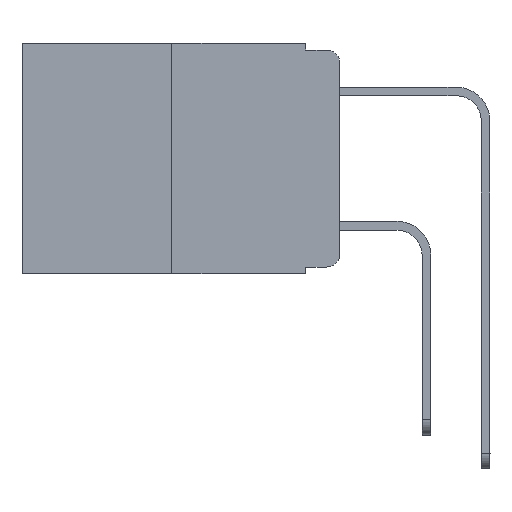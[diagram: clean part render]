
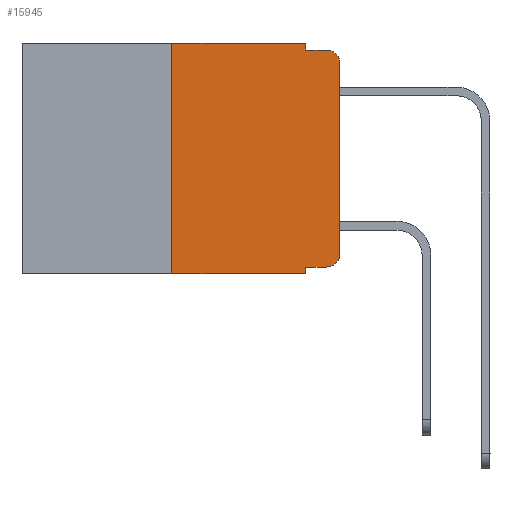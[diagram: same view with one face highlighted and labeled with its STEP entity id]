
A CAD part, left-side view. The second image highlights one B-rep face of the part: STEP entity #15945.
In plain terms, the highlighted planar face has unit normal (-1, 0, 0).
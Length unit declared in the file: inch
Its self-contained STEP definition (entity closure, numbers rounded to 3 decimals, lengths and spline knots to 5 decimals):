
#130 = VECTOR ( 'NONE', #8051, 39.37008 ) ;
#310 = ORIENTED_EDGE ( 'NONE', *, *, #6966, .T. ) ;
#363 = CARTESIAN_POINT ( 'NONE',  ( 0., 0., 0. ) ) ;
#552 = CARTESIAN_POINT ( 'NONE',  ( 0., 0.25, -0.343 ) ) ;
#640 = CARTESIAN_POINT ( 'NONE',  ( 0., 0.473, 0. ) ) ;
#662 = LINE ( 'NONE', #10816, #15736 ) ;
#1404 = VERTEX_POINT ( 'NONE', #552 ) ;
#1606 = VERTEX_POINT ( 'NONE', #12505 ) ;
#1628 = VECTOR ( 'NONE', #15412, 39.37008 ) ;
#1970 = LINE ( 'NONE', #9194, #6161 ) ;
#2006 = VERTEX_POINT ( 'NONE', #8278 ) ;
#2030 = ORIENTED_EDGE ( 'NONE', *, *, #8877, .F. ) ;
#2296 = DIRECTION ( 'NONE',  ( 1., 0., 0. ) ) ;
#2863 = ORIENTED_EDGE ( 'NONE', *, *, #17228, .F. ) ;
#2881 = VECTOR ( 'NONE', #17953, 39.37008 ) ;
#3000 = EDGE_CURVE ( 'NONE', #16953, #4364, #6071, .T. ) ;
#3018 = DIRECTION ( 'NONE',  ( 0., 0., 1. ) ) ;
#3477 = LINE ( 'NONE', #640, #3752 ) ;
#3718 = AXIS2_PLACEMENT_3D ( 'NONE', #7315, #15811, #14385 ) ;
#3752 = VECTOR ( 'NONE', #10371, 39.37008 ) ;
#3949 = VECTOR ( 'NONE', #8951, 39.37008 ) ;
#4364 = VERTEX_POINT ( 'NONE', #15149 ) ;
#4545 = CIRCLE ( 'NONE', #10470, 0.02 ) ;
#4652 = CARTESIAN_POINT ( 'NONE',  ( 0., 0.25, 0. ) ) ;
#4974 = ORIENTED_EDGE ( 'NONE', *, *, #6975, .T. ) ;
#5080 = LINE ( 'NONE', #8145, #130 ) ;
#5528 = ORIENTED_EDGE ( 'NONE', *, *, #12385, .T. ) ;
#6071 = LINE ( 'NONE', #363, #14674 ) ;
#6157 = CARTESIAN_POINT ( 'NONE',  ( 0., 0.051, -0.333 ) ) ;
#6161 = VECTOR ( 'NONE', #7621, 39.37008 ) ;
#6610 = LINE ( 'NONE', #12227, #2881 ) ;
#6828 = CARTESIAN_POINT ( 'NONE',  ( 0., 0., -0.313 ) ) ;
#6966 = EDGE_CURVE ( 'NONE', #4364, #10477, #4545, .T. ) ;
#6975 = EDGE_CURVE ( 'NONE', #1404, #7607, #5080, .T. ) ;
#7315 = CARTESIAN_POINT ( 'NONE',  ( 0., 0.02, -0.313 ) ) ;
#7607 = VERTEX_POINT ( 'NONE', #14930 ) ;
#7621 = DIRECTION ( 'NONE',  ( 0., -1., 0. ) ) ;
#8051 = DIRECTION ( 'NONE',  ( 0., -1., 0. ) ) ;
#8145 = CARTESIAN_POINT ( 'NONE',  ( 0., 0.473, -0.343 ) ) ;
#8229 = FACE_OUTER_BOUND ( 'NONE', #14494, .T. ) ;
#8278 = CARTESIAN_POINT ( 'NONE',  ( 0., 0.051, -0.01 ) ) ;
#8298 = VERTEX_POINT ( 'NONE', #16605 ) ;
#8877 = EDGE_CURVE ( 'NONE', #1606, #7607, #15326, .T. ) ;
#8951 = DIRECTION ( 'NONE',  ( 0., -1., 0. ) ) ;
#9020 = EDGE_CURVE ( 'NONE', #1606, #12892, #13046, .T. ) ;
#9194 = CARTESIAN_POINT ( 'NONE',  ( 0., 0.051, -0.01 ) ) ;
#10232 = ORIENTED_EDGE ( 'NONE', *, *, #11311, .F. ) ;
#10371 = DIRECTION ( 'NONE',  ( 0., -1., 0. ) ) ;
#10470 = AXIS2_PLACEMENT_3D ( 'NONE', #15003, #16252, #17818 ) ;
#10477 = VERTEX_POINT ( 'NONE', #16560 ) ;
#10610 = VERTEX_POINT ( 'NONE', #4652 ) ;
#10810 = PLANE ( 'NONE',  #15209 ) ;
#10816 = CARTESIAN_POINT ( 'NONE',  ( 0., 0.25, 0. ) ) ;
#11289 = ORIENTED_EDGE ( 'NONE', *, *, #17674, .F. ) ;
#11311 = EDGE_CURVE ( 'NONE', #1404, #10610, #662, .T. ) ;
#11537 = ORIENTED_EDGE ( 'NONE', *, *, #3000, .T. ) ;
#12227 = CARTESIAN_POINT ( 'NONE',  ( 0., 0.051, 0. ) ) ;
#12385 = EDGE_CURVE ( 'NONE', #12892, #16953, #16034, .T. ) ;
#12505 = CARTESIAN_POINT ( 'NONE',  ( 0., 0.051, -0.333 ) ) ;
#12892 = VERTEX_POINT ( 'NONE', #12983 ) ;
#12983 = CARTESIAN_POINT ( 'NONE',  ( 0., 0.02, -0.333 ) ) ;
#13046 = LINE ( 'NONE', #6157, #3949 ) ;
#13229 = EDGE_CURVE ( 'NONE', #8298, #2006, #6610, .T. ) ;
#14239 = CARTESIAN_POINT ( 'NONE',  ( 0., 0.051, 0. ) ) ;
#14341 = ORIENTED_EDGE ( 'NONE', *, *, #13229, .F. ) ;
#14385 = DIRECTION ( 'NONE',  ( 0., 0., -1. ) ) ;
#14494 = EDGE_LOOP ( 'NONE', ( #11537, #310, #11289, #14341, #2863, #10232, #4974, #2030, #16738, #5528 ) ) ;
#14674 = VECTOR ( 'NONE', #3018, 39.37008 ) ;
#14930 = CARTESIAN_POINT ( 'NONE',  ( 0., 0.051, -0.343 ) ) ;
#15003 = CARTESIAN_POINT ( 'NONE',  ( 0., 0.02, -0.03 ) ) ;
#15149 = CARTESIAN_POINT ( 'NONE',  ( 0., 0., -0.03 ) ) ;
#15209 = AXIS2_PLACEMENT_3D ( 'NONE', #17636, #2296, #15257 ) ;
#15257 = DIRECTION ( 'NONE',  ( 0., 0., -1. ) ) ;
#15326 = LINE ( 'NONE', #14239, #1628 ) ;
#15412 = DIRECTION ( 'NONE',  ( 0., 0., -1. ) ) ;
#15736 = VECTOR ( 'NONE', #16331, 39.37008 ) ;
#15811 = DIRECTION ( 'NONE',  ( -1., 0., 0. ) ) ;
#15945 = ADVANCED_FACE ( 'NONE', ( #8229 ), #10810, .F. ) ;
#16034 = CIRCLE ( 'NONE', #3718, 0.02 ) ;
#16252 = DIRECTION ( 'NONE',  ( -1., 0., 0. ) ) ;
#16331 = DIRECTION ( 'NONE',  ( 0., 0., 1. ) ) ;
#16560 = CARTESIAN_POINT ( 'NONE',  ( 0., 0.02, -0.01 ) ) ;
#16605 = CARTESIAN_POINT ( 'NONE',  ( 0., 0.051, 0. ) ) ;
#16738 = ORIENTED_EDGE ( 'NONE', *, *, #9020, .T. ) ;
#16953 = VERTEX_POINT ( 'NONE', #6828 ) ;
#17228 = EDGE_CURVE ( 'NONE', #10610, #8298, #3477, .T. ) ;
#17636 = CARTESIAN_POINT ( 'NONE',  ( 0., 0.473, 0. ) ) ;
#17674 = EDGE_CURVE ( 'NONE', #2006, #10477, #1970, .T. ) ;
#17818 = DIRECTION ( 'NONE',  ( 0., 0., -1. ) ) ;
#17953 = DIRECTION ( 'NONE',  ( 0., 0., -1. ) ) ;
